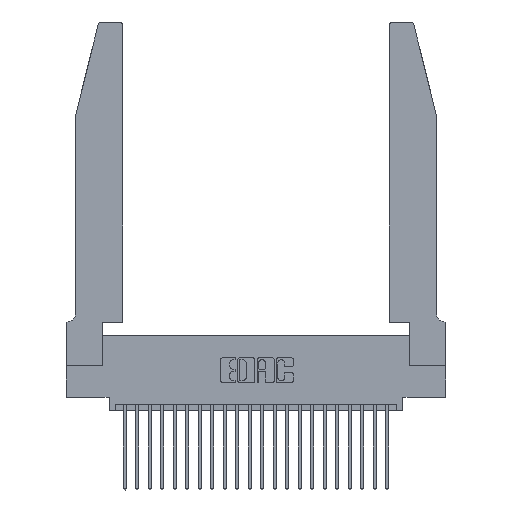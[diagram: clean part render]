
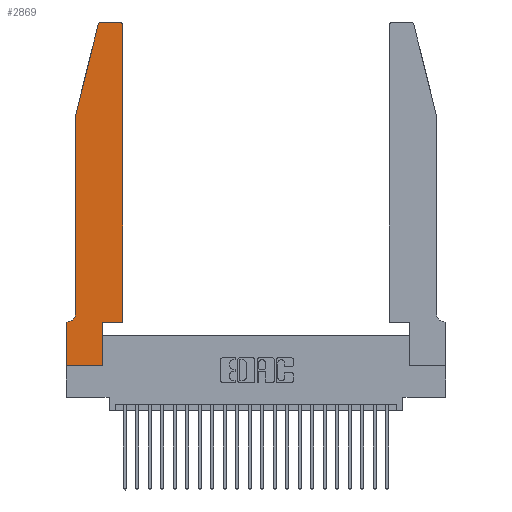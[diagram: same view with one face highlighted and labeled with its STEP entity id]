
A CAD part, top view. The second image highlights one B-rep face of the part: STEP entity #2869.
In plain terms, the highlighted planar face has unit normal (0, 0, 1).
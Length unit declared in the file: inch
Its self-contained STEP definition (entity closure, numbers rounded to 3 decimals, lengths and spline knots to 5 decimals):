
#45 = VECTOR ( 'NONE', #14222, 39.37008 ) ;
#222 = CARTESIAN_POINT ( 'NONE',  ( 0.4205, 2.72, 0.37 ) ) ;
#380 = CARTESIAN_POINT ( 'NONE',  ( 0., 0., 0.37 ) ) ;
#413 = ORIENTED_EDGE ( 'NONE', *, *, #5655, .T. ) ;
#464 = VERTEX_POINT ( 'NONE', #11095 ) ;
#550 = DIRECTION ( 'NONE',  ( 0., 0., 1. ) ) ;
#717 = EDGE_CURVE ( 'NONE', #1746, #464, #22098, .T. ) ;
#968 = ORIENTED_EDGE ( 'NONE', *, *, #22983, .T. ) ;
#1009 = EDGE_CURVE ( 'NONE', #11871, #11197, #18525, .T. ) ;
#1309 = VERTEX_POINT ( 'NONE', #18853 ) ;
#1746 = VERTEX_POINT ( 'NONE', #10947 ) ;
#1957 = EDGE_CURVE ( 'NONE', #21249, #16957, #19962, .T. ) ;
#2050 = VERTEX_POINT ( 'NONE', #11331 ) ;
#2067 = DIRECTION ( 'NONE',  ( 0., 0., 1. ) ) ;
#2154 = AXIS2_PLACEMENT_3D ( 'NONE', #13630, #7939, #23362 ) ;
#2486 = EDGE_CURVE ( 'NONE', #464, #23548, #16027, .T. ) ;
#2813 = ORIENTED_EDGE ( 'NONE', *, *, #13988, .T. ) ;
#2869 = ADVANCED_FACE ( 'NONE', ( #10235 ), #3899, .T. ) ;
#2909 = CARTESIAN_POINT ( 'NONE',  ( 0.4505, 0.35, 0.37 ) ) ;
#3899 = PLANE ( 'NONE',  #11493 ) ;
#4912 = CARTESIAN_POINT ( 'NONE',  ( 0.0755, 2., 0.37 ) ) ;
#5025 = EDGE_CURVE ( 'NONE', #10544, #21249, #20706, .T. ) ;
#5276 = ORIENTED_EDGE ( 'NONE', *, *, #20050, .T. ) ;
#5591 = VERTEX_POINT ( 'NONE', #7385 ) ;
#5655 = EDGE_CURVE ( 'NONE', #16957, #2050, #15335, .T. ) ;
#5711 = AXIS2_PLACEMENT_3D ( 'NONE', #17769, #6229, #15902 ) ;
#5912 = CARTESIAN_POINT ( 'NONE',  ( 0.284, 2.75, 0.37 ) ) ;
#6229 = DIRECTION ( 'NONE',  ( 0., 0., -1. ) ) ;
#6615 = ORIENTED_EDGE ( 'NONE', *, *, #1009, .T. ) ;
#6752 = CARTESIAN_POINT ( 'NONE',  ( 0.25487, 2.72718, 0.37 ) ) ;
#6789 = CARTESIAN_POINT ( 'NONE',  ( 0.4505, 0.35, 0.37 ) ) ;
#6811 = VECTOR ( 'NONE', #20316, 39.37008 ) ;
#7168 = CARTESIAN_POINT ( 'NONE',  ( 0.2865, 0.35, 0.37 ) ) ;
#7385 = CARTESIAN_POINT ( 'NONE',  ( 0.2865, 0., 0.37 ) ) ;
#7939 = DIRECTION ( 'NONE',  ( 0., 0., 1. ) ) ;
#8074 = EDGE_CURVE ( 'NONE', #5591, #11871, #11601, .T. ) ;
#8495 = EDGE_LOOP ( 'NONE', ( #24295, #968, #5276, #9950, #11929, #413, #19569, #2813, #14303, #6615, #17783, #11508 ) ) ;
#8613 = VECTOR ( 'NONE', #20666, 39.37008 ) ;
#8705 = LINE ( 'NONE', #2909, #45 ) ;
#8732 = VECTOR ( 'NONE', #13934, 39.37008 ) ;
#9950 = ORIENTED_EDGE ( 'NONE', *, *, #5025, .T. ) ;
#9968 = CARTESIAN_POINT ( 'NONE',  ( 0.0055, 0.35, 0.37 ) ) ;
#10235 = FACE_OUTER_BOUND ( 'NONE', #8495, .T. ) ;
#10544 = VERTEX_POINT ( 'NONE', #22587 ) ;
#10790 = VECTOR ( 'NONE', #19613, 39.37008 ) ;
#10947 = CARTESIAN_POINT ( 'NONE',  ( 0.4505, 2.72, 0.37 ) ) ;
#11095 = CARTESIAN_POINT ( 'NONE',  ( 0.4205, 2.75, 0.37 ) ) ;
#11100 = EDGE_CURVE ( 'NONE', #2050, #1309, #13231, .T. ) ;
#11197 = VERTEX_POINT ( 'NONE', #6789 ) ;
#11198 = DIRECTION ( 'NONE',  ( 1., 0., 0. ) ) ;
#11331 = CARTESIAN_POINT ( 'NONE',  ( 0., 0.35, 0.37 ) ) ;
#11493 = AXIS2_PLACEMENT_3D ( 'NONE', #21391, #2067, #17440 ) ;
#11508 = ORIENTED_EDGE ( 'NONE', *, *, #717, .T. ) ;
#11601 = LINE ( 'NONE', #14744, #6811 ) ;
#11871 = VERTEX_POINT ( 'NONE', #7168 ) ;
#11929 = ORIENTED_EDGE ( 'NONE', *, *, #1957, .T. ) ;
#12129 = LINE ( 'NONE', #14725, #14863 ) ;
#12917 = CARTESIAN_POINT ( 'NONE',  ( 0.0755, 2., 0.37 ) ) ;
#12954 = DIRECTION ( 'NONE',  ( -1., 0., 0. ) ) ;
#13201 = VECTOR ( 'NONE', #18635, 39.37008 ) ;
#13231 = LINE ( 'NONE', #380, #8732 ) ;
#13630 = CARTESIAN_POINT ( 'NONE',  ( 0.284, 2.72, 0.37 ) ) ;
#13934 = DIRECTION ( 'NONE',  ( 0., -1., 0. ) ) ;
#13937 = DIRECTION ( 'NONE',  ( 1., 0., 0. ) ) ;
#13960 = VECTOR ( 'NONE', #11198, 39.37008 ) ;
#13988 = EDGE_CURVE ( 'NONE', #1309, #5591, #12129, .T. ) ;
#14222 = DIRECTION ( 'NONE',  ( 0., 1., 0. ) ) ;
#14303 = ORIENTED_EDGE ( 'NONE', *, *, #8074, .T. ) ;
#14725 = CARTESIAN_POINT ( 'NONE',  ( 0., 0., 0.37 ) ) ;
#14744 = CARTESIAN_POINT ( 'NONE',  ( 0.2865, 0.35, 0.37 ) ) ;
#14863 = VECTOR ( 'NONE', #16692, 39.37008 ) ;
#14871 = AXIS2_PLACEMENT_3D ( 'NONE', #222, #550, #13937 ) ;
#15208 = CIRCLE ( 'NONE', #2154, 0.03 ) ;
#15335 = LINE ( 'NONE', #23235, #10790 ) ;
#15902 = DIRECTION ( 'NONE',  ( -1., 0., 0. ) ) ;
#16027 = LINE ( 'NONE', #24507, #18120 ) ;
#16692 = DIRECTION ( 'NONE',  ( 1., 0., 0. ) ) ;
#16957 = VERTEX_POINT ( 'NONE', #9968 ) ;
#17440 = DIRECTION ( 'NONE',  ( 1., 0., 0. ) ) ;
#17769 = CARTESIAN_POINT ( 'NONE',  ( 0.0055, 0.42, 0.37 ) ) ;
#17783 = ORIENTED_EDGE ( 'NONE', *, *, #20013, .T. ) ;
#18120 = VECTOR ( 'NONE', #12954, 39.37008 ) ;
#18525 = LINE ( 'NONE', #20585, #13960 ) ;
#18635 = DIRECTION ( 'NONE',  ( -0.239, -0.971, 0. ) ) ;
#18853 = CARTESIAN_POINT ( 'NONE',  ( 0., 0., 0.37 ) ) ;
#19569 = ORIENTED_EDGE ( 'NONE', *, *, #11100, .T. ) ;
#19585 = LINE ( 'NONE', #4912, #13201 ) ;
#19613 = DIRECTION ( 'NONE',  ( -1., 0., 0. ) ) ;
#19751 = CARTESIAN_POINT ( 'NONE',  ( 0.0755, 0.42, 0.37 ) ) ;
#19962 = CIRCLE ( 'NONE', #5711, 0.07 ) ;
#20013 = EDGE_CURVE ( 'NONE', #11197, #1746, #8705, .T. ) ;
#20050 = EDGE_CURVE ( 'NONE', #24645, #10544, #19585, .T. ) ;
#20316 = DIRECTION ( 'NONE',  ( 0., 1., 0. ) ) ;
#20585 = CARTESIAN_POINT ( 'NONE',  ( 0.4505, 0.35, 0.37 ) ) ;
#20666 = DIRECTION ( 'NONE',  ( 0., -1., 0. ) ) ;
#20706 = LINE ( 'NONE', #12917, #8613 ) ;
#21249 = VERTEX_POINT ( 'NONE', #19751 ) ;
#21391 = CARTESIAN_POINT ( 'NONE',  ( 0., 0.35, 0.37 ) ) ;
#22098 = CIRCLE ( 'NONE', #14871, 0.03 ) ;
#22587 = CARTESIAN_POINT ( 'NONE',  ( 0.0755, 2., 0.37 ) ) ;
#22983 = EDGE_CURVE ( 'NONE', #23548, #24645, #15208, .T. ) ;
#23235 = CARTESIAN_POINT ( 'NONE',  ( 0.0755, 0.35, 0.37 ) ) ;
#23362 = DIRECTION ( 'NONE',  ( 1., 0., 0. ) ) ;
#23548 = VERTEX_POINT ( 'NONE', #5912 ) ;
#24295 = ORIENTED_EDGE ( 'NONE', *, *, #2486, .T. ) ;
#24507 = CARTESIAN_POINT ( 'NONE',  ( 0.2605, 2.75, 0.37 ) ) ;
#24645 = VERTEX_POINT ( 'NONE', #6752 ) ;
